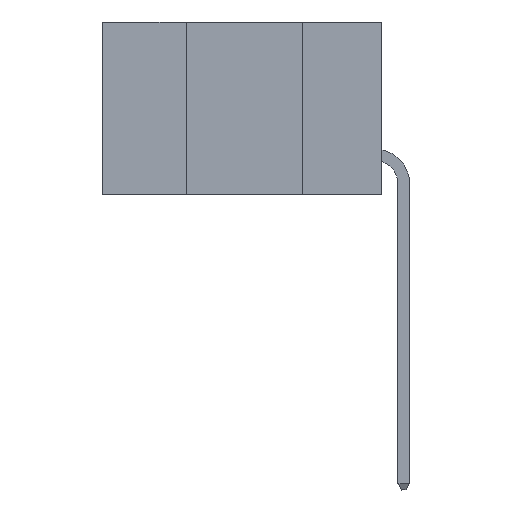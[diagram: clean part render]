
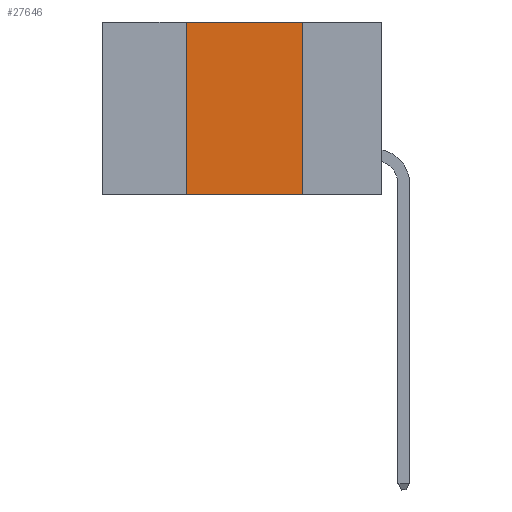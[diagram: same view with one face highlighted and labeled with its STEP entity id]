
A CAD part, left-side view. The second image highlights one B-rep face of the part: STEP entity #27646.
In plain terms, the highlighted planar face has unit normal (-1, 0, 0).
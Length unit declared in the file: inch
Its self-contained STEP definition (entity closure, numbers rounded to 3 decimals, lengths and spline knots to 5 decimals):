
#1334 = CARTESIAN_POINT ( 'NONE',  ( 0., 0.6, 0. ) ) ;
#4499 = DIRECTION ( 'NONE',  ( 0., 0., -1. ) ) ;
#4974 = VECTOR ( 'NONE', #25169, 39.37008 ) ;
#5926 = CARTESIAN_POINT ( 'NONE',  ( 0., 0.6, -0.37 ) ) ;
#6047 = ORIENTED_EDGE ( 'NONE', *, *, #39598, .F. ) ;
#6575 = CARTESIAN_POINT ( 'NONE',  ( 0., 0.42, 0. ) ) ;
#8015 = ORIENTED_EDGE ( 'NONE', *, *, #11048, .F. ) ;
#8838 = AXIS2_PLACEMENT_3D ( 'NONE', #1334, #23191, #4499 ) ;
#9707 = CARTESIAN_POINT ( 'NONE',  ( 0., 0.17, 0. ) ) ;
#11048 = EDGE_CURVE ( 'NONE', #32852, #15249, #14121, .T. ) ;
#11109 = VERTEX_POINT ( 'NONE', #19523 ) ;
#12035 = EDGE_CURVE ( 'NONE', #11109, #32852, #38944, .T. ) ;
#13443 = ORIENTED_EDGE ( 'NONE', *, *, #31471, .T. ) ;
#14121 = LINE ( 'NONE', #15595, #18029 ) ;
#14137 = CARTESIAN_POINT ( 'NONE',  ( 0., 0.42, 0. ) ) ;
#14545 = VECTOR ( 'NONE', #29294, 39.37008 ) ;
#15249 = VERTEX_POINT ( 'NONE', #38496 ) ;
#15595 = CARTESIAN_POINT ( 'NONE',  ( 0., 0.6, 0. ) ) ;
#18029 = VECTOR ( 'NONE', #18573, 39.37008 ) ;
#18573 = DIRECTION ( 'NONE',  ( 0., -1., 0. ) ) ;
#19523 = CARTESIAN_POINT ( 'NONE',  ( 0., 0.42, -0.37 ) ) ;
#20056 = PLANE ( 'NONE',  #8838 ) ;
#21206 = DIRECTION ( 'NONE',  ( 0., -1., 0. ) ) ;
#23191 = DIRECTION ( 'NONE',  ( 1., 0., 0. ) ) ;
#25169 = DIRECTION ( 'NONE',  ( 0., 0., -1. ) ) ;
#25666 = EDGE_LOOP ( 'NONE', ( #6047, #8015, #38291, #13443 ) ) ;
#27646 = ADVANCED_FACE ( 'NONE', ( #29675 ), #20056, .F. ) ;
#29294 = DIRECTION ( 'NONE',  ( 0., 0., 1. ) ) ;
#29312 = VERTEX_POINT ( 'NONE', #39415 ) ;
#29675 = FACE_OUTER_BOUND ( 'NONE', #25666, .T. ) ;
#31471 = EDGE_CURVE ( 'NONE', #11109, #29312, #34142, .T. ) ;
#32852 = VERTEX_POINT ( 'NONE', #6575 ) ;
#34142 = LINE ( 'NONE', #5926, #35608 ) ;
#34754 = LINE ( 'NONE', #9707, #4974 ) ;
#35608 = VECTOR ( 'NONE', #21206, 39.37008 ) ;
#38291 = ORIENTED_EDGE ( 'NONE', *, *, #12035, .F. ) ;
#38496 = CARTESIAN_POINT ( 'NONE',  ( 0., 0.17, 0. ) ) ;
#38944 = LINE ( 'NONE', #14137, #14545 ) ;
#39415 = CARTESIAN_POINT ( 'NONE',  ( 0., 0.17, -0.37 ) ) ;
#39598 = EDGE_CURVE ( 'NONE', #15249, #29312, #34754, .T. ) ;
